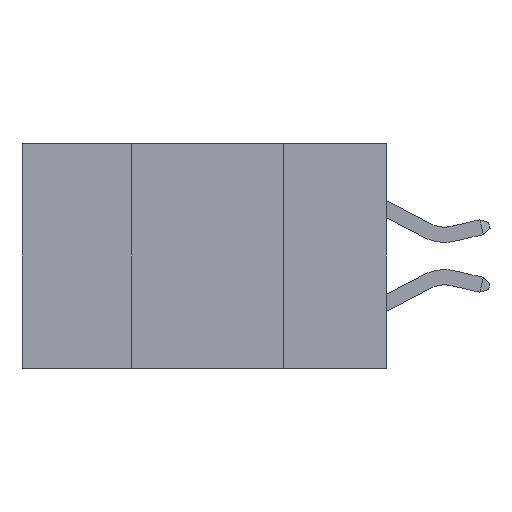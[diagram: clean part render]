
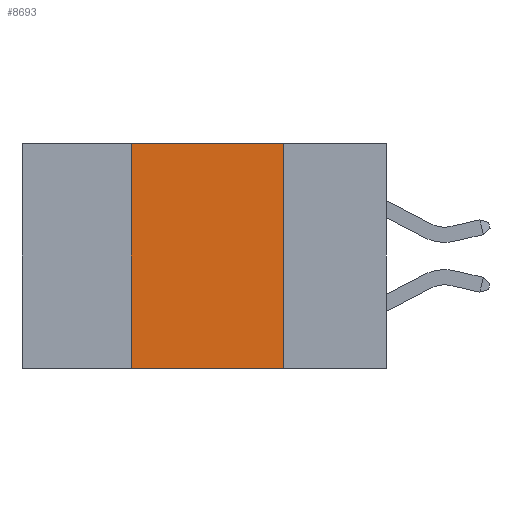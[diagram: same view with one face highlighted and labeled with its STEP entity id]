
A CAD part, left-side view. The second image highlights one B-rep face of the part: STEP entity #8693.
In plain terms, the highlighted planar face has unit normal (-1, 0, 0).
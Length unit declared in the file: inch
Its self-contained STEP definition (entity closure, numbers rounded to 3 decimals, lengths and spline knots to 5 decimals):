
#2373 = VECTOR ( 'NONE', #12158, 39.37008 ) ;
#2517 = FACE_OUTER_BOUND ( 'NONE', #16954, .T. ) ;
#2724 = DIRECTION ( 'NONE',  ( 1., 0., 0. ) ) ;
#2841 = CARTESIAN_POINT ( 'NONE',  ( 0., 0.6, 0. ) ) ;
#2882 = VERTEX_POINT ( 'NONE', #18727 ) ;
#3973 = VECTOR ( 'NONE', #19110, 39.37008 ) ;
#4078 = EDGE_CURVE ( 'NONE', #9227, #2882, #17847, .T. ) ;
#4243 = CARTESIAN_POINT ( 'NONE',  ( 0., 0.17, -0.37 ) ) ;
#4597 = VERTEX_POINT ( 'NONE', #16623 ) ;
#5249 = AXIS2_PLACEMENT_3D ( 'NONE', #2841, #2724, #6072 ) ;
#5578 = EDGE_CURVE ( 'NONE', #9227, #12937, #15574, .T. ) ;
#6072 = DIRECTION ( 'NONE',  ( 0., 0., -1. ) ) ;
#6427 = ORIENTED_EDGE ( 'NONE', *, *, #4078, .F. ) ;
#7858 = DIRECTION ( 'NONE',  ( 0., 0., 1. ) ) ;
#8693 = ADVANCED_FACE ( 'NONE', ( #2517 ), #17584, .F. ) ;
#9110 = VECTOR ( 'NONE', #7858, 39.37008 ) ;
#9227 = VERTEX_POINT ( 'NONE', #19584 ) ;
#9775 = CARTESIAN_POINT ( 'NONE',  ( 0., 0.42, -0.37 ) ) ;
#10491 = DIRECTION ( 'NONE',  ( 0., -1., 0. ) ) ;
#10619 = CARTESIAN_POINT ( 'NONE',  ( 0., 0.6, -0.37 ) ) ;
#12158 = DIRECTION ( 'NONE',  ( 0., 0., -1. ) ) ;
#12468 = CARTESIAN_POINT ( 'NONE',  ( 0., 0.17, -0.37 ) ) ;
#12762 = EDGE_CURVE ( 'NONE', #2882, #4597, #13388, .T. ) ;
#12937 = VERTEX_POINT ( 'NONE', #4243 ) ;
#13388 = LINE ( 'NONE', #19955, #14409 ) ;
#13771 = EDGE_CURVE ( 'NONE', #4597, #12937, #20335, .T. ) ;
#14409 = VECTOR ( 'NONE', #10491, 39.37008 ) ;
#15152 = ORIENTED_EDGE ( 'NONE', *, *, #5578, .T. ) ;
#15574 = LINE ( 'NONE', #10619, #3973 ) ;
#16623 = CARTESIAN_POINT ( 'NONE',  ( 0., 0.17, 0. ) ) ;
#16954 = EDGE_LOOP ( 'NONE', ( #19359, #18854, #6427, #15152 ) ) ;
#17584 = PLANE ( 'NONE',  #5249 ) ;
#17847 = LINE ( 'NONE', #9775, #9110 ) ;
#18727 = CARTESIAN_POINT ( 'NONE',  ( 0., 0.42, 0. ) ) ;
#18854 = ORIENTED_EDGE ( 'NONE', *, *, #12762, .F. ) ;
#19110 = DIRECTION ( 'NONE',  ( 0., -1., 0. ) ) ;
#19359 = ORIENTED_EDGE ( 'NONE', *, *, #13771, .F. ) ;
#19584 = CARTESIAN_POINT ( 'NONE',  ( 0., 0.42, -0.37 ) ) ;
#19955 = CARTESIAN_POINT ( 'NONE',  ( 0., 0.6, 0. ) ) ;
#20335 = LINE ( 'NONE', #12468, #2373 ) ;
